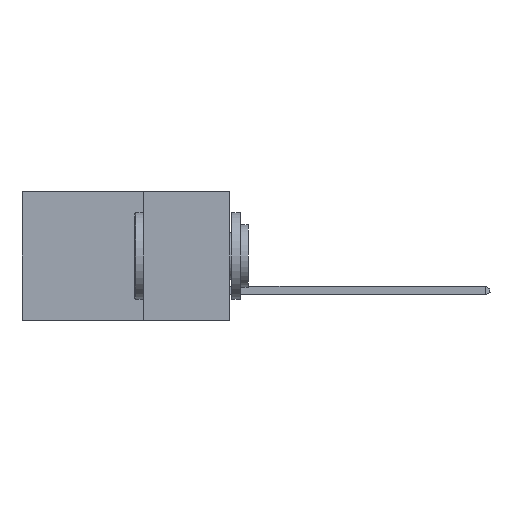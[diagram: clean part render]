
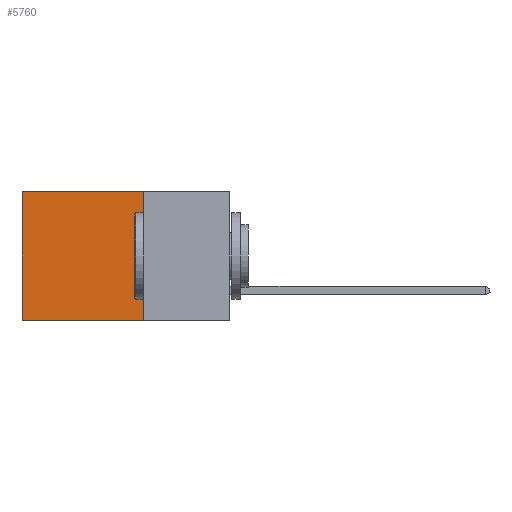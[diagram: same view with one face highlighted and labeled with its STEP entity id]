
A CAD part, left-side view. The second image highlights one B-rep face of the part: STEP entity #5760.
In plain terms, the highlighted planar face has unit normal (-1, 0, 0).
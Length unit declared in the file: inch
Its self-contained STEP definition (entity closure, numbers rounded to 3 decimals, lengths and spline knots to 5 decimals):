
#22 = DIRECTION ( 'NONE',  ( 1., 0., 0. ) ) ;
#118 = DIRECTION ( 'NONE',  ( 0., 0., -1. ) ) ;
#121 = VERTEX_POINT ( 'NONE', #6917 ) ;
#158 = FACE_OUTER_BOUND ( 'NONE', #7079, .T. ) ;
#226 = VECTOR ( 'NONE', #6149, 39.37008 ) ;
#298 = CARTESIAN_POINT ( 'NONE',  ( 0.298, 0.25, 0. ) ) ;
#373 = EDGE_CURVE ( 'NONE', #6653, #121, #9322, .T. ) ;
#1171 = VERTEX_POINT ( 'NONE', #7565 ) ;
#1256 = CARTESIAN_POINT ( 'NONE',  ( 0.298, 0.6, -0.37 ) ) ;
#1391 = ORIENTED_EDGE ( 'NONE', *, *, #6825, .T. ) ;
#1431 = CARTESIAN_POINT ( 'NONE',  ( 0.298, 0.25, 0. ) ) ;
#1503 = ORIENTED_EDGE ( 'NONE', *, *, #373, .F. ) ;
#1585 = EDGE_CURVE ( 'NONE', #121, #8734, #8154, .T. ) ;
#2514 = CARTESIAN_POINT ( 'NONE',  ( 0.298, 0.25, 0. ) ) ;
#2919 = CARTESIAN_POINT ( 'NONE',  ( 0.298, 0.25, -0.37 ) ) ;
#3078 = VECTOR ( 'NONE', #6419, 39.37008 ) ;
#3230 = DIRECTION ( 'NONE',  ( 0., 0., -1. ) ) ;
#3414 = VECTOR ( 'NONE', #10498, 39.37008 ) ;
#3481 = CARTESIAN_POINT ( 'NONE',  ( 0.298, 0.6, 0. ) ) ;
#4575 = ORIENTED_EDGE ( 'NONE', *, *, #6307, .T. ) ;
#4966 = PLANE ( 'NONE',  #8005 ) ;
#5431 = VECTOR ( 'NONE', #118, 39.37008 ) ;
#5760 = ADVANCED_FACE ( 'NONE', ( #158 ), #4966, .F. ) ;
#6149 = DIRECTION ( 'NONE',  ( 0., 1., 0. ) ) ;
#6307 = EDGE_CURVE ( 'NONE', #1171, #8734, #6751, .T. ) ;
#6419 = DIRECTION ( 'NONE',  ( 0., 1., 0. ) ) ;
#6653 = VERTEX_POINT ( 'NONE', #298 ) ;
#6751 = LINE ( 'NONE', #3481, #5431 ) ;
#6825 = EDGE_CURVE ( 'NONE', #6653, #1171, #8172, .T. ) ;
#6917 = CARTESIAN_POINT ( 'NONE',  ( 0.298, 0.25, -0.37 ) ) ;
#7079 = EDGE_LOOP ( 'NONE', ( #4575, #9017, #1503, #1391 ) ) ;
#7565 = CARTESIAN_POINT ( 'NONE',  ( 0.298, 0.6, 0. ) ) ;
#8005 = AXIS2_PLACEMENT_3D ( 'NONE', #2514, #22, #3230 ) ;
#8034 = CARTESIAN_POINT ( 'NONE',  ( 0.298, 0.25, 0. ) ) ;
#8154 = LINE ( 'NONE', #2919, #226 ) ;
#8172 = LINE ( 'NONE', #1431, #3078 ) ;
#8734 = VERTEX_POINT ( 'NONE', #1256 ) ;
#9017 = ORIENTED_EDGE ( 'NONE', *, *, #1585, .F. ) ;
#9322 = LINE ( 'NONE', #8034, #3414 ) ;
#10498 = DIRECTION ( 'NONE',  ( 0., 0., -1. ) ) ;
